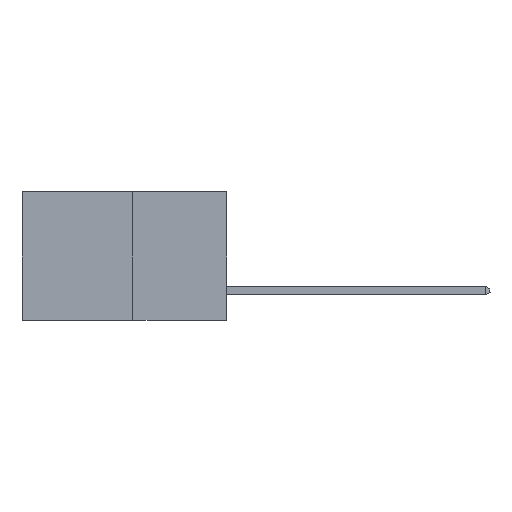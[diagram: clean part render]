
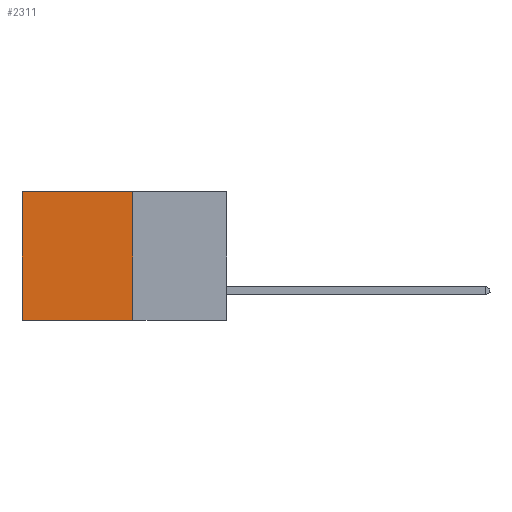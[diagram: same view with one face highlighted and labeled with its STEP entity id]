
A CAD part, left-side view. The second image highlights one B-rep face of the part: STEP entity #2311.
In plain terms, the highlighted planar face has unit normal (-1, 0, 0).
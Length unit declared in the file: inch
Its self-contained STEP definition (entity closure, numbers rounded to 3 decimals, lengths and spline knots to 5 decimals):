
#1248 = VERTEX_POINT ( 'NONE', #10434 ) ;
#1554 = AXIS2_PLACEMENT_3D ( 'NONE', #14670, #14623, #16472 ) ;
#1829 = EDGE_CURVE ( 'NONE', #20358, #1248, #7437, .T. ) ;
#2201 = VERTEX_POINT ( 'NONE', #19304 ) ;
#2311 = ADVANCED_FACE ( 'NONE', ( #2585 ), #4551, .F. ) ;
#2585 = FACE_OUTER_BOUND ( 'NONE', #16094, .T. ) ;
#3110 = VECTOR ( 'NONE', #7045, 39.37008 ) ;
#3675 = VECTOR ( 'NONE', #6519, 39.37008 ) ;
#4551 = PLANE ( 'NONE',  #1554 ) ;
#4904 = CARTESIAN_POINT ( 'NONE',  ( 0.277, 0.27, -0.37 ) ) ;
#4953 = ORIENTED_EDGE ( 'NONE', *, *, #7459, .F. ) ;
#5435 = CARTESIAN_POINT ( 'NONE',  ( 0.277, 0.27, 0. ) ) ;
#5844 = CARTESIAN_POINT ( 'NONE',  ( 0.277, 0.59, -0.37 ) ) ;
#5863 = ORIENTED_EDGE ( 'NONE', *, *, #1829, .T. ) ;
#6519 = DIRECTION ( 'NONE',  ( 0., 0., -1. ) ) ;
#7045 = DIRECTION ( 'NONE',  ( 0., 1., 0. ) ) ;
#7426 = LINE ( 'NONE', #5435, #3110 ) ;
#7437 = LINE ( 'NONE', #5844, #12735 ) ;
#7459 = EDGE_CURVE ( 'NONE', #13428, #1248, #8059, .T. ) ;
#7765 = ORIENTED_EDGE ( 'NONE', *, *, #17559, .F. ) ;
#8059 = LINE ( 'NONE', #10836, #11829 ) ;
#10434 = CARTESIAN_POINT ( 'NONE',  ( 0.277, 0.59, -0.37 ) ) ;
#10836 = CARTESIAN_POINT ( 'NONE',  ( 0.277, 0.27, -0.37 ) ) ;
#11829 = VECTOR ( 'NONE', #13368, 39.37008 ) ;
#12735 = VECTOR ( 'NONE', #17391, 39.37008 ) ;
#12760 = LINE ( 'NONE', #4904, #3675 ) ;
#13231 = ORIENTED_EDGE ( 'NONE', *, *, #18436, .T. ) ;
#13368 = DIRECTION ( 'NONE',  ( 0., 1., 0. ) ) ;
#13428 = VERTEX_POINT ( 'NONE', #20570 ) ;
#13491 = CARTESIAN_POINT ( 'NONE',  ( 0.277, 0.59, 0. ) ) ;
#14623 = DIRECTION ( 'NONE',  ( 1., 0., 0. ) ) ;
#14670 = CARTESIAN_POINT ( 'NONE',  ( 0.277, 0.27, -0.37 ) ) ;
#16094 = EDGE_LOOP ( 'NONE', ( #5863, #4953, #7765, #13231 ) ) ;
#16472 = DIRECTION ( 'NONE',  ( 0., 0., -1. ) ) ;
#17391 = DIRECTION ( 'NONE',  ( 0., 0., -1. ) ) ;
#17559 = EDGE_CURVE ( 'NONE', #2201, #13428, #12760, .T. ) ;
#18436 = EDGE_CURVE ( 'NONE', #2201, #20358, #7426, .T. ) ;
#19304 = CARTESIAN_POINT ( 'NONE',  ( 0.277, 0.27, 0. ) ) ;
#20358 = VERTEX_POINT ( 'NONE', #13491 ) ;
#20570 = CARTESIAN_POINT ( 'NONE',  ( 0.277, 0.27, -0.37 ) ) ;
